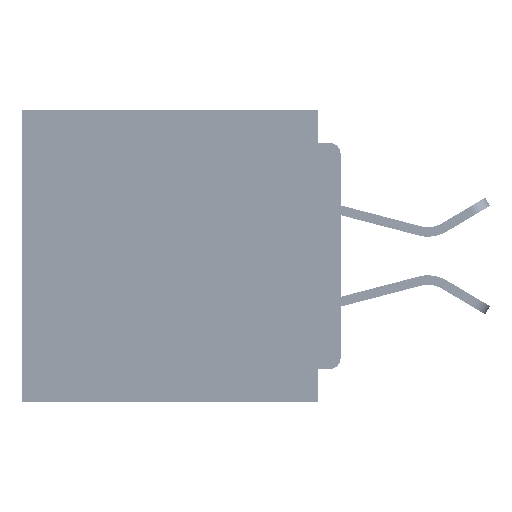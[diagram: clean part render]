
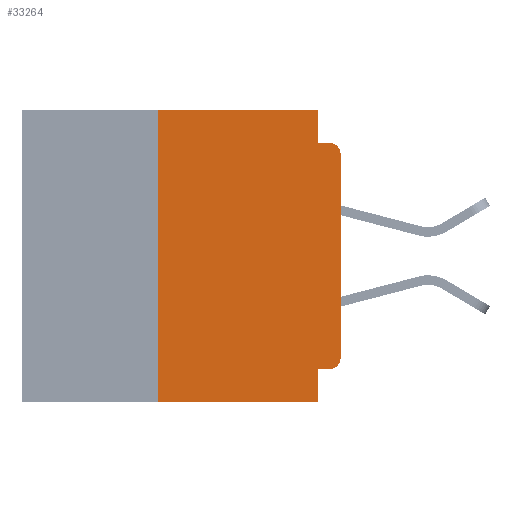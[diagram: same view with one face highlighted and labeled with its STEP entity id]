
A CAD part, left-side view. The second image highlights one B-rep face of the part: STEP entity #33264.
In plain terms, the highlighted planar face has unit normal (-1, 0, 0).
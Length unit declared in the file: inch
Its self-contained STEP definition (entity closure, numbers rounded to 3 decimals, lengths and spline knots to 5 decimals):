
#192 = VECTOR ( 'NONE', #7033, 39.37008 ) ;
#1312 = EDGE_CURVE ( 'NONE', #36619, #62932, #6338, .T. ) ;
#2001 = DIRECTION ( 'NONE',  ( 0., 0., 1. ) ) ;
#2902 = CARTESIAN_POINT ( 'NONE',  ( 0., 0., -0.045 ) ) ;
#3449 = LINE ( 'NONE', #42977, #192 ) ;
#3632 = CARTESIAN_POINT ( 'NONE',  ( 0., 0.015, -0.06 ) ) ;
#4293 = LINE ( 'NONE', #4888, #17972 ) ;
#4376 = ORIENTED_EDGE ( 'NONE', *, *, #64338, .F. ) ;
#4703 = CARTESIAN_POINT ( 'NONE',  ( 0., 0.437, 0. ) ) ;
#4888 = CARTESIAN_POINT ( 'NONE',  ( 0., 0.031, 0. ) ) ;
#4958 = CARTESIAN_POINT ( 'NONE',  ( 0., 0.031, -0.4 ) ) ;
#6338 = LINE ( 'NONE', #10770, #57683 ) ;
#7033 = DIRECTION ( 'NONE',  ( 0., 1., 0. ) ) ;
#7113 = VERTEX_POINT ( 'NONE', #31401 ) ;
#7458 = ORIENTED_EDGE ( 'NONE', *, *, #18433, .T. ) ;
#8091 = DIRECTION ( 'NONE',  ( 0., -1., 0. ) ) ;
#8799 = LINE ( 'NONE', #2902, #34544 ) ;
#8821 = DIRECTION ( 'NONE',  ( 0., 0., -1. ) ) ;
#8951 = VERTEX_POINT ( 'NONE', #16787 ) ;
#10770 = CARTESIAN_POINT ( 'NONE',  ( 0., 0.031, -0.4 ) ) ;
#10898 = VECTOR ( 'NONE', #26762, 39.37008 ) ;
#11614 = VERTEX_POINT ( 'NONE', #30096 ) ;
#12638 = CARTESIAN_POINT ( 'NONE',  ( 0., 0.015, -0.34 ) ) ;
#15069 = VERTEX_POINT ( 'NONE', #22261 ) ;
#15265 = VERTEX_POINT ( 'NONE', #44267 ) ;
#15752 = CARTESIAN_POINT ( 'NONE',  ( 0., 0.25, -0.4 ) ) ;
#15996 = AXIS2_PLACEMENT_3D ( 'NONE', #4703, #61194, #30561 ) ;
#16412 = LINE ( 'NONE', #38020, #45335 ) ;
#16787 = CARTESIAN_POINT ( 'NONE',  ( 0., 0., -0.06 ) ) ;
#16841 = VECTOR ( 'NONE', #40820, 39.37008 ) ;
#17273 = CIRCLE ( 'NONE', #63742, 0.015 ) ;
#17795 = CARTESIAN_POINT ( 'NONE',  ( 0., 0.015, -0.355 ) ) ;
#17821 = DIRECTION ( 'NONE',  ( 0., 0., -1. ) ) ;
#17972 = VECTOR ( 'NONE', #40854, 39.37008 ) ;
#18433 = EDGE_CURVE ( 'NONE', #8951, #15265, #17273, .T. ) ;
#19257 = AXIS2_PLACEMENT_3D ( 'NONE', #12638, #48545, #17821 ) ;
#22081 = EDGE_CURVE ( 'NONE', #39701, #7113, #66429, .T. ) ;
#22261 = CARTESIAN_POINT ( 'NONE',  ( 0., 0.031, -0.045 ) ) ;
#24255 = VERTEX_POINT ( 'NONE', #58037 ) ;
#25501 = CARTESIAN_POINT ( 'NONE',  ( 0., 0.437, -0.4 ) ) ;
#26762 = DIRECTION ( 'NONE',  ( 0., -1., 0. ) ) ;
#27275 = CARTESIAN_POINT ( 'NONE',  ( 0., 0.25, -0.4 ) ) ;
#30096 = CARTESIAN_POINT ( 'NONE',  ( 0., 0., -0.34 ) ) ;
#30561 = DIRECTION ( 'NONE',  ( 0., 0., -1. ) ) ;
#31004 = ORIENTED_EDGE ( 'NONE', *, *, #44922, .F. ) ;
#31401 = CARTESIAN_POINT ( 'NONE',  ( 0., 0.25, 0. ) ) ;
#31494 = CIRCLE ( 'NONE', #19257, 0.015 ) ;
#33264 = ADVANCED_FACE ( 'NONE', ( #43699 ), #56067, .F. ) ;
#34544 = VECTOR ( 'NONE', #8091, 39.37008 ) ;
#35744 = EDGE_CURVE ( 'NONE', #39701, #62932, #45772, .T. ) ;
#36619 = VERTEX_POINT ( 'NONE', #60435 ) ;
#36926 = CARTESIAN_POINT ( 'NONE',  ( 0., 0.437, 0. ) ) ;
#38020 = CARTESIAN_POINT ( 'NONE',  ( 0., 0., 0. ) ) ;
#39614 = DIRECTION ( 'NONE',  ( -1., 0., 0. ) ) ;
#39701 = VERTEX_POINT ( 'NONE', #15752 ) ;
#40251 = ORIENTED_EDGE ( 'NONE', *, *, #65600, .F. ) ;
#40820 = DIRECTION ( 'NONE',  ( 0., -1., 0. ) ) ;
#40854 = DIRECTION ( 'NONE',  ( 0., 0., -1. ) ) ;
#42977 = CARTESIAN_POINT ( 'NONE',  ( 0., 0., -0.355 ) ) ;
#43699 = FACE_OUTER_BOUND ( 'NONE', #50926, .T. ) ;
#43983 = ORIENTED_EDGE ( 'NONE', *, *, #54327, .F. ) ;
#44267 = CARTESIAN_POINT ( 'NONE',  ( 0., 0.015, -0.045 ) ) ;
#44922 = EDGE_CURVE ( 'NONE', #24255, #15069, #4293, .T. ) ;
#45335 = VECTOR ( 'NONE', #2001, 39.37008 ) ;
#45772 = LINE ( 'NONE', #25501, #16841 ) ;
#46696 = DIRECTION ( 'NONE',  ( 0., 0., -1. ) ) ;
#47752 = ORIENTED_EDGE ( 'NONE', *, *, #1312, .F. ) ;
#48545 = DIRECTION ( 'NONE',  ( -1., 0., 0. ) ) ;
#49980 = EDGE_CURVE ( 'NONE', #11614, #8951, #16412, .T. ) ;
#50926 = EDGE_LOOP ( 'NONE', ( #55391, #7458, #43983, #31004, #4376, #62321, #62140, #47752, #40251, #51763 ) ) ;
#51268 = EDGE_CURVE ( 'NONE', #66202, #11614, #31494, .T. ) ;
#51763 = ORIENTED_EDGE ( 'NONE', *, *, #51268, .T. ) ;
#51819 = LINE ( 'NONE', #36926, #10898 ) ;
#52834 = VECTOR ( 'NONE', #63105, 39.37008 ) ;
#54327 = EDGE_CURVE ( 'NONE', #15069, #15265, #8799, .T. ) ;
#55391 = ORIENTED_EDGE ( 'NONE', *, *, #49980, .T. ) ;
#56067 = PLANE ( 'NONE',  #15996 ) ;
#57683 = VECTOR ( 'NONE', #46696, 39.37008 ) ;
#58037 = CARTESIAN_POINT ( 'NONE',  ( 0., 0.031, 0. ) ) ;
#60435 = CARTESIAN_POINT ( 'NONE',  ( 0., 0.031, -0.355 ) ) ;
#61194 = DIRECTION ( 'NONE',  ( 1., 0., 0. ) ) ;
#62140 = ORIENTED_EDGE ( 'NONE', *, *, #35744, .T. ) ;
#62321 = ORIENTED_EDGE ( 'NONE', *, *, #22081, .F. ) ;
#62932 = VERTEX_POINT ( 'NONE', #4958 ) ;
#63105 = DIRECTION ( 'NONE',  ( 0., 0., 1. ) ) ;
#63742 = AXIS2_PLACEMENT_3D ( 'NONE', #3632, #39614, #8821 ) ;
#64338 = EDGE_CURVE ( 'NONE', #7113, #24255, #51819, .T. ) ;
#65600 = EDGE_CURVE ( 'NONE', #66202, #36619, #3449, .T. ) ;
#66202 = VERTEX_POINT ( 'NONE', #17795 ) ;
#66429 = LINE ( 'NONE', #27275, #52834 ) ;
